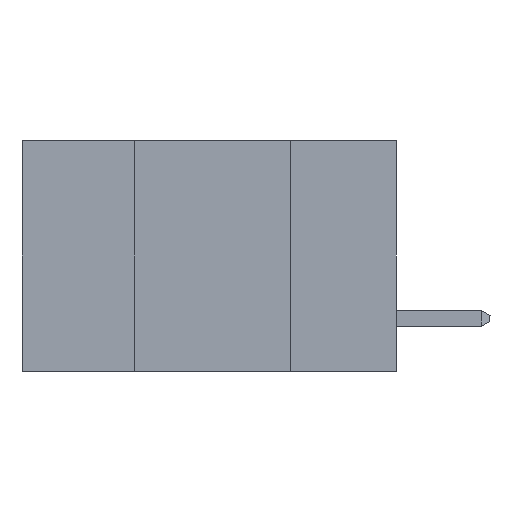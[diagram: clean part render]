
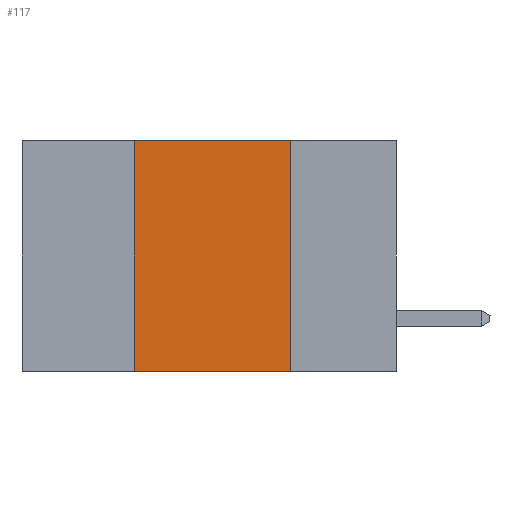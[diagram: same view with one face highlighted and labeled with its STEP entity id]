
A CAD part, left-side view. The second image highlights one B-rep face of the part: STEP entity #117.
In plain terms, the highlighted planar face has unit normal (-1, 0, 0).
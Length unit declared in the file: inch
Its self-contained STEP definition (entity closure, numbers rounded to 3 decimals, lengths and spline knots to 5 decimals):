
#117 = ADVANCED_FACE ( 'NONE', ( #1148 ), #13544, .F. ) ;
#786 = DIRECTION ( 'NONE',  ( 0., -1., 0. ) ) ;
#835 = EDGE_LOOP ( 'NONE', ( #5876, #7863, #8702, #5379 ) ) ;
#1148 = FACE_OUTER_BOUND ( 'NONE', #835, .T. ) ;
#1532 = EDGE_CURVE ( 'NONE', #13289, #7612, #4945, .T. ) ;
#2195 = DIRECTION ( 'NONE',  ( 1., 0., 0. ) ) ;
#2461 = LINE ( 'NONE', #12693, #4556 ) ;
#3111 = VECTOR ( 'NONE', #9590, 39.37008 ) ;
#3489 = VERTEX_POINT ( 'NONE', #14261 ) ;
#3877 = VERTEX_POINT ( 'NONE', #12082 ) ;
#4556 = VECTOR ( 'NONE', #14650, 39.37008 ) ;
#4869 = CARTESIAN_POINT ( 'NONE',  ( 0., 0.6, -0.37 ) ) ;
#4945 = LINE ( 'NONE', #4869, #3111 ) ;
#5261 = CARTESIAN_POINT ( 'NONE',  ( 0., 0.42, -0.37 ) ) ;
#5352 = AXIS2_PLACEMENT_3D ( 'NONE', #7890, #2195, #10198 ) ;
#5379 = ORIENTED_EDGE ( 'NONE', *, *, #1532, .T. ) ;
#5802 = CARTESIAN_POINT ( 'NONE',  ( 0., 0.42, -0.37 ) ) ;
#5876 = ORIENTED_EDGE ( 'NONE', *, *, #6171, .F. ) ;
#6171 = EDGE_CURVE ( 'NONE', #3877, #7612, #2461, .T. ) ;
#6565 = VECTOR ( 'NONE', #786, 39.37008 ) ;
#6612 = CARTESIAN_POINT ( 'NONE',  ( 0., 0.6, 0. ) ) ;
#7257 = CARTESIAN_POINT ( 'NONE',  ( 0., 0.17, -0.37 ) ) ;
#7612 = VERTEX_POINT ( 'NONE', #7257 ) ;
#7863 = ORIENTED_EDGE ( 'NONE', *, *, #10824, .F. ) ;
#7890 = CARTESIAN_POINT ( 'NONE',  ( 0., 0.6, 0. ) ) ;
#8702 = ORIENTED_EDGE ( 'NONE', *, *, #10814, .F. ) ;
#9590 = DIRECTION ( 'NONE',  ( 0., -1., 0. ) ) ;
#9916 = VECTOR ( 'NONE', #11170, 39.37008 ) ;
#10198 = DIRECTION ( 'NONE',  ( 0., 0., -1. ) ) ;
#10814 = EDGE_CURVE ( 'NONE', #13289, #3489, #12125, .T. ) ;
#10824 = EDGE_CURVE ( 'NONE', #3489, #3877, #11025, .T. ) ;
#11025 = LINE ( 'NONE', #6612, #6565 ) ;
#11170 = DIRECTION ( 'NONE',  ( 0., 0., 1. ) ) ;
#12082 = CARTESIAN_POINT ( 'NONE',  ( 0., 0.17, 0. ) ) ;
#12125 = LINE ( 'NONE', #5261, #9916 ) ;
#12693 = CARTESIAN_POINT ( 'NONE',  ( 0., 0.17, -0.37 ) ) ;
#13289 = VERTEX_POINT ( 'NONE', #5802 ) ;
#13544 = PLANE ( 'NONE',  #5352 ) ;
#14261 = CARTESIAN_POINT ( 'NONE',  ( 0., 0.42, 0. ) ) ;
#14650 = DIRECTION ( 'NONE',  ( 0., 0., -1. ) ) ;
